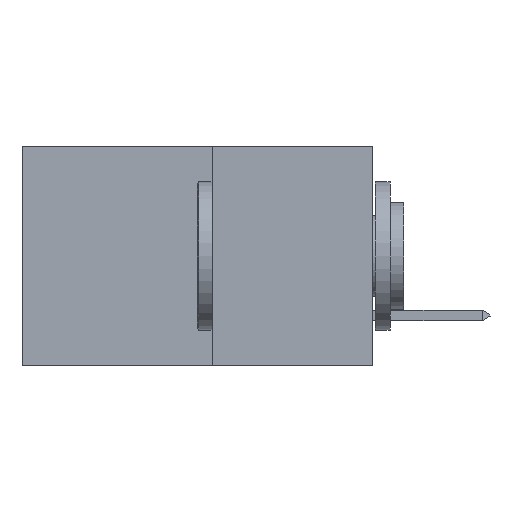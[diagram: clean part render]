
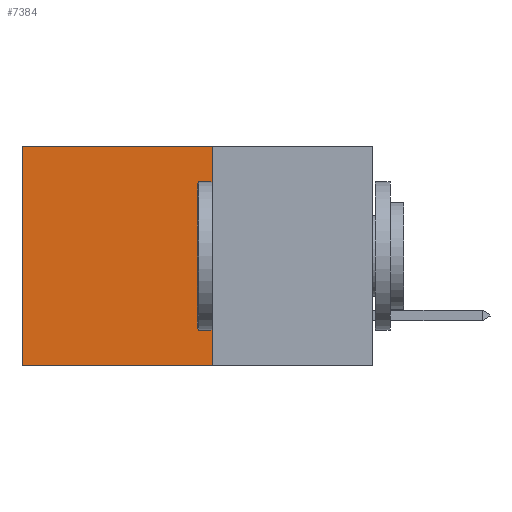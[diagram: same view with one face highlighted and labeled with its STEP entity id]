
A CAD part, left-side view. The second image highlights one B-rep face of the part: STEP entity #7384.
In plain terms, the highlighted planar face has unit normal (-1, 0, 0).
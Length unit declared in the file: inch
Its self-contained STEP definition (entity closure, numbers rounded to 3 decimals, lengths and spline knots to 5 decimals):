
#1293 = DIRECTION ( 'NONE',  ( 0., 0., -1. ) ) ;
#2102 = CARTESIAN_POINT ( 'NONE',  ( 0.277, 0.59, -0.37 ) ) ;
#2871 = CARTESIAN_POINT ( 'NONE',  ( 0.277, 0.27, -0.37 ) ) ;
#2947 = ORIENTED_EDGE ( 'NONE', *, *, #17866, .F. ) ;
#3012 = VECTOR ( 'NONE', #31155, 39.37008 ) ;
#3443 = CARTESIAN_POINT ( 'NONE',  ( 0.277, 0.27, -0.37 ) ) ;
#5200 = VERTEX_POINT ( 'NONE', #5718 ) ;
#5580 = ORIENTED_EDGE ( 'NONE', *, *, #11799, .T. ) ;
#5718 = CARTESIAN_POINT ( 'NONE',  ( 0.277, 0.27, 0. ) ) ;
#6293 = DIRECTION ( 'NONE',  ( 1., 0., 0. ) ) ;
#6603 = CARTESIAN_POINT ( 'NONE',  ( 0.277, 0.59, -0.37 ) ) ;
#6638 = DIRECTION ( 'NONE',  ( 0., 0., -1. ) ) ;
#6724 = VECTOR ( 'NONE', #21342, 39.37008 ) ;
#7240 = VERTEX_POINT ( 'NONE', #3443 ) ;
#7384 = ADVANCED_FACE ( 'NONE', ( #14056 ), #29391, .F. ) ;
#9201 = CARTESIAN_POINT ( 'NONE',  ( 0.277, 0.59, 0. ) ) ;
#9364 = DIRECTION ( 'NONE',  ( 0., 1., 0. ) ) ;
#9371 = CARTESIAN_POINT ( 'NONE',  ( 0.277, 0.27, 0. ) ) ;
#10331 = EDGE_CURVE ( 'NONE', #23675, #23017, #20242, .T. ) ;
#10536 = CARTESIAN_POINT ( 'NONE',  ( 0.277, 0.27, -0.37 ) ) ;
#11799 = EDGE_CURVE ( 'NONE', #5200, #23675, #28681, .T. ) ;
#13418 = VECTOR ( 'NONE', #6638, 39.37008 ) ;
#14056 = FACE_OUTER_BOUND ( 'NONE', #16634, .T. ) ;
#15054 = ORIENTED_EDGE ( 'NONE', *, *, #10331, .T. ) ;
#16634 = EDGE_LOOP ( 'NONE', ( #15054, #22566, #2947, #5580 ) ) ;
#16748 = LINE ( 'NONE', #10536, #3012 ) ;
#17866 = EDGE_CURVE ( 'NONE', #5200, #7240, #16748, .T. ) ;
#18820 = CARTESIAN_POINT ( 'NONE',  ( 0.277, 0.27, -0.37 ) ) ;
#20242 = LINE ( 'NONE', #2102, #13418 ) ;
#20455 = LINE ( 'NONE', #18820, #6724 ) ;
#21342 = DIRECTION ( 'NONE',  ( 0., 1., 0. ) ) ;
#22566 = ORIENTED_EDGE ( 'NONE', *, *, #26096, .F. ) ;
#23017 = VERTEX_POINT ( 'NONE', #6603 ) ;
#23675 = VERTEX_POINT ( 'NONE', #9201 ) ;
#26096 = EDGE_CURVE ( 'NONE', #7240, #23017, #20455, .T. ) ;
#28681 = LINE ( 'NONE', #9371, #29486 ) ;
#29391 = PLANE ( 'NONE',  #31514 ) ;
#29486 = VECTOR ( 'NONE', #9364, 39.37008 ) ;
#31155 = DIRECTION ( 'NONE',  ( 0., 0., -1. ) ) ;
#31514 = AXIS2_PLACEMENT_3D ( 'NONE', #2871, #6293, #1293 ) ;
